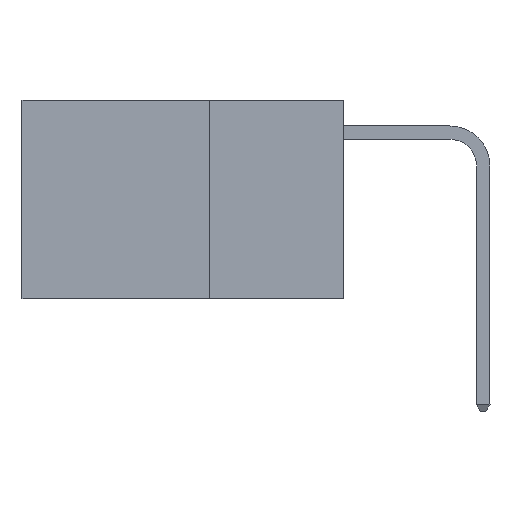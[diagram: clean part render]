
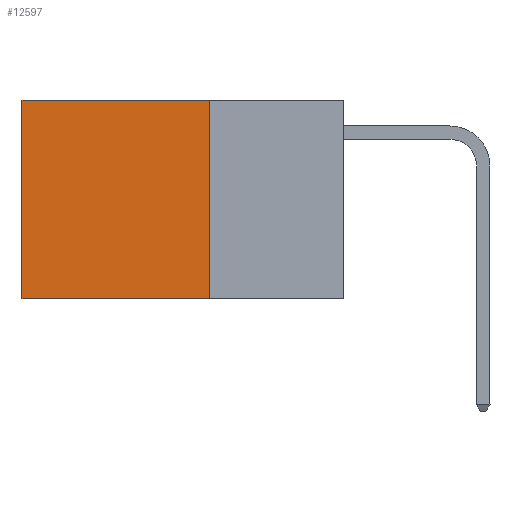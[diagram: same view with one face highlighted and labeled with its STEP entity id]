
A CAD part, left-side view. The second image highlights one B-rep face of the part: STEP entity #12597.
In plain terms, the highlighted planar face has unit normal (-1, 0, 0).
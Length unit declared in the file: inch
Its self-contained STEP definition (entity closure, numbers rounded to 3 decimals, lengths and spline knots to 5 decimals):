
#241 = CARTESIAN_POINT ( 'NONE',  ( 0.2625, 0.25, 0. ) ) ;
#492 = CARTESIAN_POINT ( 'NONE',  ( 0.2625, 0.6, 0. ) ) ;
#1028 = EDGE_CURVE ( 'NONE', #13994, #13746, #17212, .T. ) ;
#1222 = LINE ( 'NONE', #1565, #8610 ) ;
#1539 = VECTOR ( 'NONE', #7709, 39.37008 ) ;
#1565 = CARTESIAN_POINT ( 'NONE',  ( 0.2625, 0.25, 0. ) ) ;
#1662 = DIRECTION ( 'NONE',  ( 0., 0., -1. ) ) ;
#2206 = EDGE_LOOP ( 'NONE', ( #17605, #18695, #16662, #8725 ) ) ;
#3510 = EDGE_CURVE ( 'NONE', #12981, #13994, #1222, .T. ) ;
#4066 = VECTOR ( 'NONE', #13714, 39.37008 ) ;
#4571 = CARTESIAN_POINT ( 'NONE',  ( 0.2625, 0.6, -0.37 ) ) ;
#4686 = VERTEX_POINT ( 'NONE', #7105 ) ;
#5456 = EDGE_CURVE ( 'NONE', #12981, #4686, #9691, .T. ) ;
#5807 = VECTOR ( 'NONE', #9116, 39.37008 ) ;
#6052 = DIRECTION ( 'NONE',  ( 0., 0., -1. ) ) ;
#7105 = CARTESIAN_POINT ( 'NONE',  ( 0.2625, 0.6, 0. ) ) ;
#7435 = CARTESIAN_POINT ( 'NONE',  ( 0.2625, 0.25, 0. ) ) ;
#7709 = DIRECTION ( 'NONE',  ( 0., 1., 0. ) ) ;
#8125 = CARTESIAN_POINT ( 'NONE',  ( 0.2625, 0.25, -0.37 ) ) ;
#8610 = VECTOR ( 'NONE', #1662, 39.37008 ) ;
#8665 = FACE_OUTER_BOUND ( 'NONE', #2206, .T. ) ;
#8725 = ORIENTED_EDGE ( 'NONE', *, *, #5456, .T. ) ;
#9116 = DIRECTION ( 'NONE',  ( 0., 1., 0. ) ) ;
#9488 = CARTESIAN_POINT ( 'NONE',  ( 0.2625, 0.25, -0.37 ) ) ;
#9691 = LINE ( 'NONE', #241, #5807 ) ;
#10422 = PLANE ( 'NONE',  #13921 ) ;
#12597 = ADVANCED_FACE ( 'NONE', ( #8665 ), #10422, .F. ) ;
#12981 = VERTEX_POINT ( 'NONE', #17460 ) ;
#13275 = EDGE_CURVE ( 'NONE', #4686, #13746, #15310, .T. ) ;
#13714 = DIRECTION ( 'NONE',  ( 0., 0., -1. ) ) ;
#13746 = VERTEX_POINT ( 'NONE', #4571 ) ;
#13921 = AXIS2_PLACEMENT_3D ( 'NONE', #7435, #14854, #6052 ) ;
#13994 = VERTEX_POINT ( 'NONE', #9488 ) ;
#14854 = DIRECTION ( 'NONE',  ( 1., 0., 0. ) ) ;
#15310 = LINE ( 'NONE', #492, #4066 ) ;
#16662 = ORIENTED_EDGE ( 'NONE', *, *, #3510, .F. ) ;
#17212 = LINE ( 'NONE', #8125, #1539 ) ;
#17460 = CARTESIAN_POINT ( 'NONE',  ( 0.2625, 0.25, 0. ) ) ;
#17605 = ORIENTED_EDGE ( 'NONE', *, *, #13275, .T. ) ;
#18695 = ORIENTED_EDGE ( 'NONE', *, *, #1028, .F. ) ;
